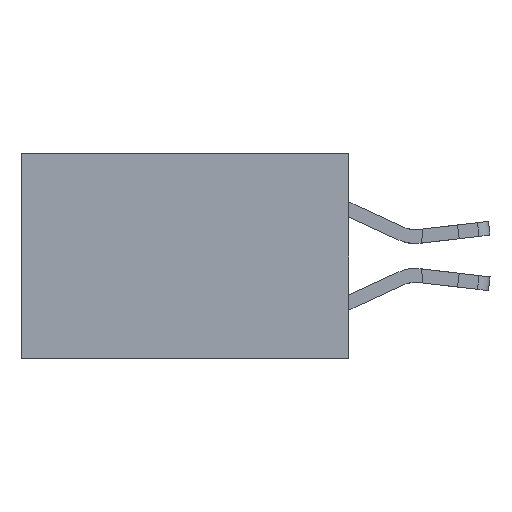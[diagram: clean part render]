
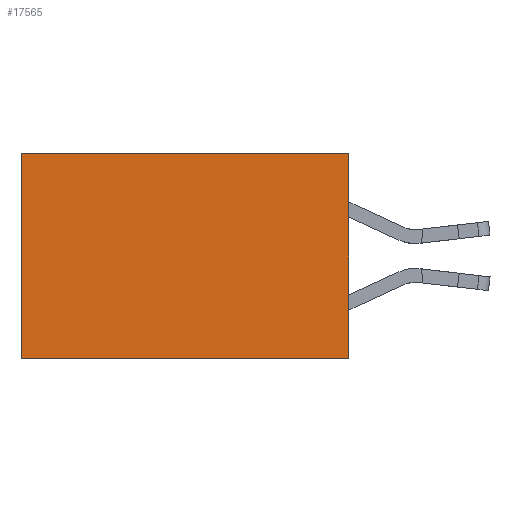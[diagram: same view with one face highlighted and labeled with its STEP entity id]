
A CAD part, left-side view. The second image highlights one B-rep face of the part: STEP entity #17565.
In plain terms, the highlighted planar face has unit normal (-1, 0, 0).
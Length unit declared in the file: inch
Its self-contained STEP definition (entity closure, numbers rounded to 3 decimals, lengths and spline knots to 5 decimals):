
#679 = EDGE_CURVE ( 'NONE', #25880, #4956, #1622, .T. ) ;
#1209 = CARTESIAN_POINT ( 'NONE',  ( 0.277, 0.59, -0.37 ) ) ;
#1622 = LINE ( 'NONE', #13161, #18171 ) ;
#1975 = PLANE ( 'NONE',  #10960 ) ;
#2945 = ORIENTED_EDGE ( 'NONE', *, *, #12842, .T. ) ;
#4183 = DIRECTION ( 'NONE',  ( 1., 0., 0. ) ) ;
#4470 = ORIENTED_EDGE ( 'NONE', *, *, #679, .F. ) ;
#4956 = VERTEX_POINT ( 'NONE', #26223 ) ;
#5959 = DIRECTION ( 'NONE',  ( 0., 1., 0. ) ) ;
#6453 = CARTESIAN_POINT ( 'NONE',  ( 0.277, 0.59, 0. ) ) ;
#6484 = FACE_OUTER_BOUND ( 'NONE', #18433, .T. ) ;
#10059 = VECTOR ( 'NONE', #27229, 39.37008 ) ;
#10125 = DIRECTION ( 'NONE',  ( 0., 0., -1. ) ) ;
#10650 = CARTESIAN_POINT ( 'NONE',  ( 0.277, 0., -0.37 ) ) ;
#10960 = AXIS2_PLACEMENT_3D ( 'NONE', #10650, #4183, #19236 ) ;
#12842 = EDGE_CURVE ( 'NONE', #24243, #14067, #22546, .T. ) ;
#13161 = CARTESIAN_POINT ( 'NONE',  ( 0.277, 0., -0.37 ) ) ;
#14067 = VERTEX_POINT ( 'NONE', #1209 ) ;
#14089 = ORIENTED_EDGE ( 'NONE', *, *, #27222, .T. ) ;
#16433 = CARTESIAN_POINT ( 'NONE',  ( 0.277, 0., 0. ) ) ;
#17022 = VECTOR ( 'NONE', #10125, 39.37008 ) ;
#17280 = DIRECTION ( 'NONE',  ( 0., 0., -1. ) ) ;
#17348 = VECTOR ( 'NONE', #5959, 39.37008 ) ;
#17565 = ADVANCED_FACE ( 'NONE', ( #6484 ), #1975, .F. ) ;
#17790 = LINE ( 'NONE', #19006, #10059 ) ;
#18171 = VECTOR ( 'NONE', #17280, 39.37008 ) ;
#18433 = EDGE_LOOP ( 'NONE', ( #2945, #24099, #4470, #14089 ) ) ;
#18852 = CARTESIAN_POINT ( 'NONE',  ( 0.277, 0., -0.37 ) ) ;
#19006 = CARTESIAN_POINT ( 'NONE',  ( 0.277, 0., 0. ) ) ;
#19236 = DIRECTION ( 'NONE',  ( 0., 0., -1. ) ) ;
#22383 = EDGE_CURVE ( 'NONE', #4956, #14067, #23494, .T. ) ;
#22546 = LINE ( 'NONE', #26803, #17022 ) ;
#23494 = LINE ( 'NONE', #18852, #17348 ) ;
#24099 = ORIENTED_EDGE ( 'NONE', *, *, #22383, .F. ) ;
#24243 = VERTEX_POINT ( 'NONE', #6453 ) ;
#25880 = VERTEX_POINT ( 'NONE', #16433 ) ;
#26223 = CARTESIAN_POINT ( 'NONE',  ( 0.277, 0., -0.37 ) ) ;
#26803 = CARTESIAN_POINT ( 'NONE',  ( 0.277, 0.59, -0.37 ) ) ;
#27222 = EDGE_CURVE ( 'NONE', #25880, #24243, #17790, .T. ) ;
#27229 = DIRECTION ( 'NONE',  ( 0., 1., 0. ) ) ;
